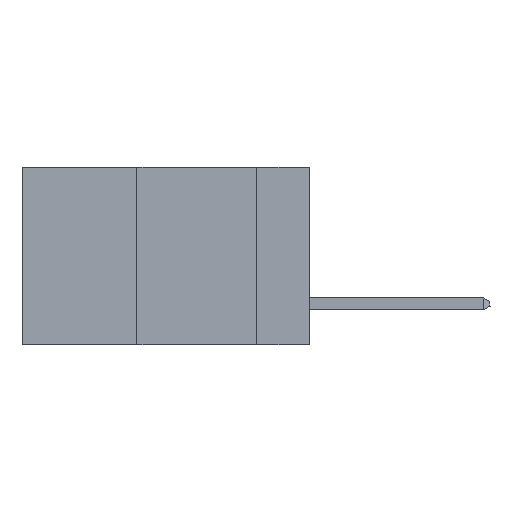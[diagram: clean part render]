
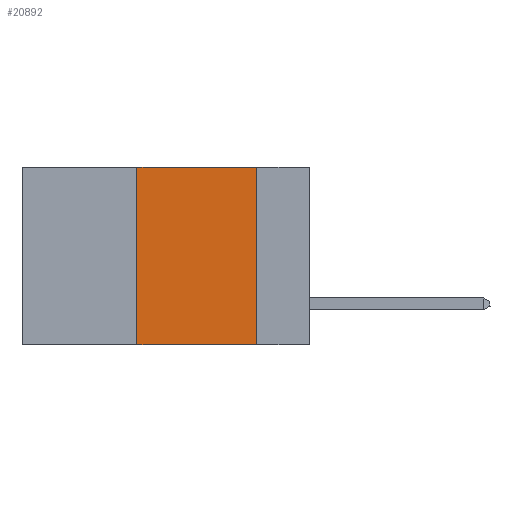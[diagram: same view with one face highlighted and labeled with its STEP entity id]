
A CAD part, left-side view. The second image highlights one B-rep face of the part: STEP entity #20892.
In plain terms, the highlighted planar face has unit normal (-1, 0, 0).
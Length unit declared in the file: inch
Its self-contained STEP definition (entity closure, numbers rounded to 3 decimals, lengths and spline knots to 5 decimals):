
#217 = EDGE_CURVE ( 'NONE', #10383, #27916, #17260, .T. ) ;
#380 = VECTOR ( 'NONE', #9053, 39.37008 ) ;
#1582 = EDGE_CURVE ( 'NONE', #27916, #7660, #5700, .T. ) ;
#2977 = EDGE_CURVE ( 'NONE', #11956, #10383, #6787, .T. ) ;
#4391 = CARTESIAN_POINT ( 'NONE',  ( 0., 0.36, 0. ) ) ;
#5205 = FACE_OUTER_BOUND ( 'NONE', #27487, .T. ) ;
#5700 = LINE ( 'NONE', #23108, #13218 ) ;
#6196 = DIRECTION ( 'NONE',  ( 0., 0., -1. ) ) ;
#6787 = LINE ( 'NONE', #25897, #380 ) ;
#7660 = VERTEX_POINT ( 'NONE', #17679 ) ;
#9051 = CARTESIAN_POINT ( 'NONE',  ( 0., 0.6, -0.37 ) ) ;
#9053 = DIRECTION ( 'NONE',  ( 0., 0., 1. ) ) ;
#9157 = EDGE_CURVE ( 'NONE', #11956, #7660, #28405, .T. ) ;
#10383 = VERTEX_POINT ( 'NONE', #4391 ) ;
#11487 = DIRECTION ( 'NONE',  ( 0., -1., 0. ) ) ;
#11741 = CARTESIAN_POINT ( 'NONE',  ( 0., 0.6, 0. ) ) ;
#11956 = VERTEX_POINT ( 'NONE', #17804 ) ;
#13218 = VECTOR ( 'NONE', #6196, 39.37008 ) ;
#13819 = DIRECTION ( 'NONE',  ( 0., 0., -1. ) ) ;
#16037 = CARTESIAN_POINT ( 'NONE',  ( 0., 0.6, 0. ) ) ;
#17128 = VECTOR ( 'NONE', #11487, 39.37008 ) ;
#17260 = LINE ( 'NONE', #11741, #30439 ) ;
#17679 = CARTESIAN_POINT ( 'NONE',  ( 0., 0.11, -0.37 ) ) ;
#17804 = CARTESIAN_POINT ( 'NONE',  ( 0., 0.36, -0.37 ) ) ;
#18070 = CARTESIAN_POINT ( 'NONE',  ( 0., 0.11, 0. ) ) ;
#18715 = ORIENTED_EDGE ( 'NONE', *, *, #2977, .F. ) ;
#20892 = ADVANCED_FACE ( 'NONE', ( #5205 ), #23397, .F. ) ;
#23108 = CARTESIAN_POINT ( 'NONE',  ( 0., 0.11, 0. ) ) ;
#23397 = PLANE ( 'NONE',  #30998 ) ;
#24046 = DIRECTION ( 'NONE',  ( 0., -1., 0. ) ) ;
#24582 = ORIENTED_EDGE ( 'NONE', *, *, #9157, .T. ) ;
#25897 = CARTESIAN_POINT ( 'NONE',  ( 0., 0.36, 0. ) ) ;
#27487 = EDGE_LOOP ( 'NONE', ( #28036, #28238, #18715, #24582 ) ) ;
#27916 = VERTEX_POINT ( 'NONE', #18070 ) ;
#28036 = ORIENTED_EDGE ( 'NONE', *, *, #1582, .F. ) ;
#28194 = DIRECTION ( 'NONE',  ( 1., 0., 0. ) ) ;
#28238 = ORIENTED_EDGE ( 'NONE', *, *, #217, .F. ) ;
#28405 = LINE ( 'NONE', #9051, #17128 ) ;
#30439 = VECTOR ( 'NONE', #24046, 39.37008 ) ;
#30998 = AXIS2_PLACEMENT_3D ( 'NONE', #16037, #28194, #13819 ) ;
